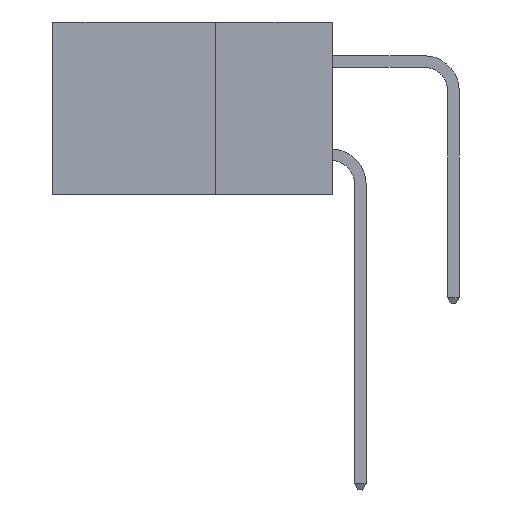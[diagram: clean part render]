
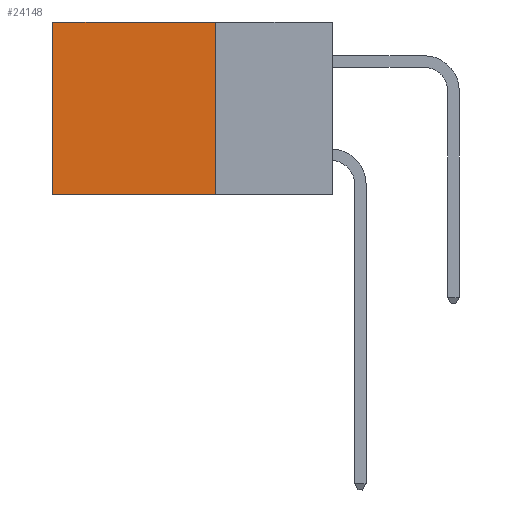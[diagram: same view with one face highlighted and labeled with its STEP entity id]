
A CAD part, left-side view. The second image highlights one B-rep face of the part: STEP entity #24148.
In plain terms, the highlighted planar face has unit normal (-1, 0, 0).
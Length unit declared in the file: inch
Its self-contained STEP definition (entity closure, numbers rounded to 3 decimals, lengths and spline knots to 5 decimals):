
#395 = ORIENTED_EDGE ( 'NONE', *, *, #28812, .F. ) ;
#757 = ORIENTED_EDGE ( 'NONE', *, *, #17358, .F. ) ;
#1073 = VECTOR ( 'NONE', #17368, 39.37008 ) ;
#1191 = CARTESIAN_POINT ( 'NONE',  ( 0.298, 0.25, -0.37 ) ) ;
#3426 = VERTEX_POINT ( 'NONE', #30198 ) ;
#4055 = CARTESIAN_POINT ( 'NONE',  ( 0.298, 0.25, 0. ) ) ;
#5298 = LINE ( 'NONE', #8560, #6743 ) ;
#5325 = VERTEX_POINT ( 'NONE', #5627 ) ;
#5627 = CARTESIAN_POINT ( 'NONE',  ( 0.298, 0.6, -0.37 ) ) ;
#5940 = VECTOR ( 'NONE', #22417, 39.37008 ) ;
#6660 = LINE ( 'NONE', #12948, #5940 ) ;
#6743 = VECTOR ( 'NONE', #11217, 39.37008 ) ;
#7909 = CARTESIAN_POINT ( 'NONE',  ( 0.298, 0.25, 0. ) ) ;
#8560 = CARTESIAN_POINT ( 'NONE',  ( 0.298, 0.25, 0. ) ) ;
#11217 = DIRECTION ( 'NONE',  ( 0., 0., -1. ) ) ;
#12382 = AXIS2_PLACEMENT_3D ( 'NONE', #27678, #14115, #14431 ) ;
#12824 = PLANE ( 'NONE',  #12382 ) ;
#12948 = CARTESIAN_POINT ( 'NONE',  ( 0.298, 0.6, 0. ) ) ;
#13589 = LINE ( 'NONE', #1191, #1073 ) ;
#13808 = DIRECTION ( 'NONE',  ( 0., 1., 0. ) ) ;
#14115 = DIRECTION ( 'NONE',  ( 1., 0., 0. ) ) ;
#14431 = DIRECTION ( 'NONE',  ( 0., 0., -1. ) ) ;
#14694 = EDGE_CURVE ( 'NONE', #27050, #27971, #29794, .T. ) ;
#15892 = EDGE_CURVE ( 'NONE', #27971, #5325, #6660, .T. ) ;
#17358 = EDGE_CURVE ( 'NONE', #27050, #3426, #5298, .T. ) ;
#17368 = DIRECTION ( 'NONE',  ( 0., 1., 0. ) ) ;
#19375 = EDGE_LOOP ( 'NONE', ( #21856, #395, #757, #24672 ) ) ;
#20884 = FACE_OUTER_BOUND ( 'NONE', #19375, .T. ) ;
#21856 = ORIENTED_EDGE ( 'NONE', *, *, #15892, .T. ) ;
#22417 = DIRECTION ( 'NONE',  ( 0., 0., -1. ) ) ;
#23188 = CARTESIAN_POINT ( 'NONE',  ( 0.298, 0.6, 0. ) ) ;
#24148 = ADVANCED_FACE ( 'NONE', ( #20884 ), #12824, .F. ) ;
#24672 = ORIENTED_EDGE ( 'NONE', *, *, #14694, .T. ) ;
#26165 = VECTOR ( 'NONE', #13808, 39.37008 ) ;
#27050 = VERTEX_POINT ( 'NONE', #7909 ) ;
#27678 = CARTESIAN_POINT ( 'NONE',  ( 0.298, 0.25, 0. ) ) ;
#27971 = VERTEX_POINT ( 'NONE', #23188 ) ;
#28812 = EDGE_CURVE ( 'NONE', #3426, #5325, #13589, .T. ) ;
#29794 = LINE ( 'NONE', #4055, #26165 ) ;
#30198 = CARTESIAN_POINT ( 'NONE',  ( 0.298, 0.25, -0.37 ) ) ;
